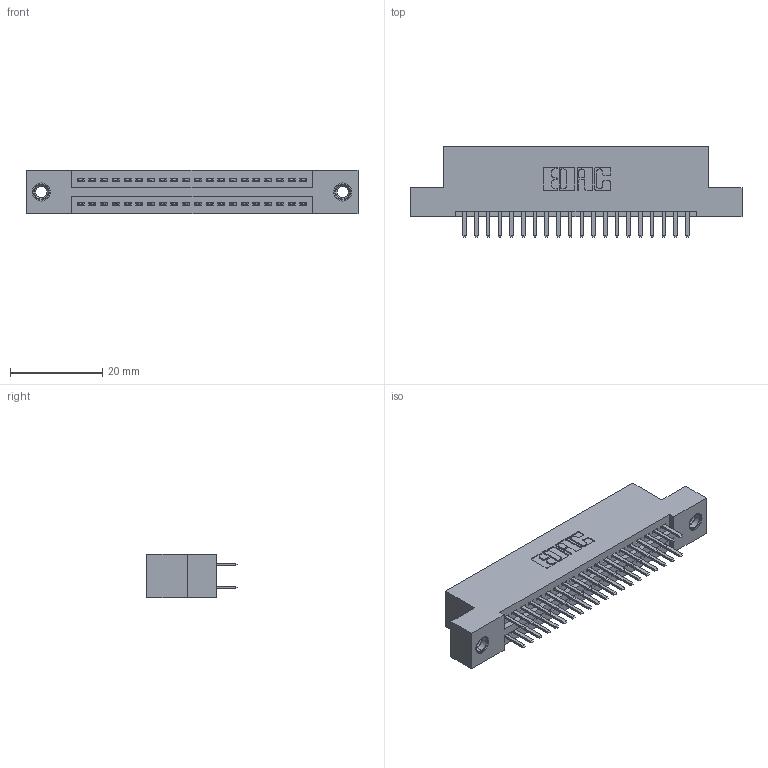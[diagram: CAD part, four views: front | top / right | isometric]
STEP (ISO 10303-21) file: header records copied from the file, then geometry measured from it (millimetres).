
FILE_DESCRIPTION (( 'STEP AP203' ), '1' );
FILE_NAME ('345-040-520-207.STEP', '2018-09-05T00:56:20', ( '' ), ( '' ), 'SwSTEP 2.0', 'SolidWorks 2016', '' );
FILE_SCHEMA (( 'CONFIG_CONTROL_DESIGN' ));
Length unit declared in the file: inch
Products named in the file (4): 345-250-001_345-250-005-103; 345-040-520-207; 345 Part_Flush Mounting Lugs - 0.156 Dia-TI; 345-292-001_345-293-120
Assembly tree (43 placements, depth 2):
  345-040-520-207
    345 Part_Flush Mounting Lugs - 0.156 Dia-TI
    345-292-001_345-293-120  x40
    345-250-001_345-250-005-103  x2
Bounding box: 72.01 x 19.68 x 9.4 mm (x, y, z)
Volume: 6759.7 mm3; surface area: 9556.4 mm2
Topology: 43 solids, 43 shells, 2346 faces, 6757 edges, 4390 vertices
Faces by surface type: plane 1512, cylinder 818, cone 12, torus 4
Entity records: 19954 total; most frequent: CARTESIAN_POINT 3359, ORIENTED_EDGE 3274, DIRECTION 3003, EDGE_CURVE 1637, LINE 1401, VECTOR 1401, VERTEX_POINT 1084, AXIS2_PLACEMENT_3D 801
